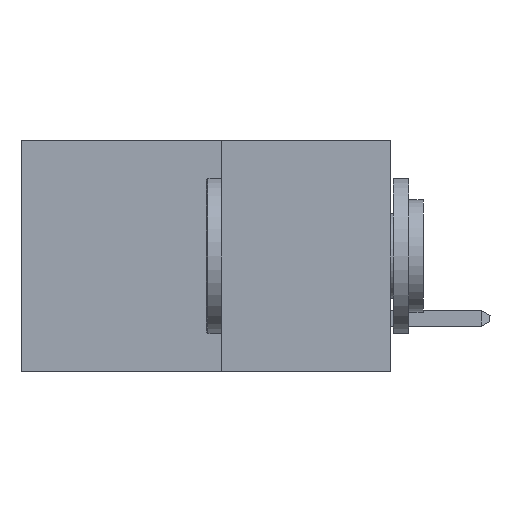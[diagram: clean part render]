
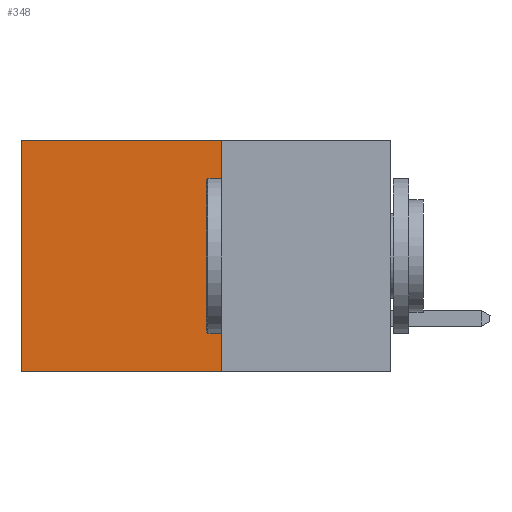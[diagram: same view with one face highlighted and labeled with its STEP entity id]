
A CAD part, left-side view. The second image highlights one B-rep face of the part: STEP entity #348.
In plain terms, the highlighted planar face has unit normal (-1, 0, 0).
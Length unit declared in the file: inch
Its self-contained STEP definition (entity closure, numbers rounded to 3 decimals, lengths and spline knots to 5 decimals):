
#348 = ADVANCED_FACE ( 'NONE', ( #4977 ), #7914, .F. ) ;
#482 = DIRECTION ( 'NONE',  ( 0., 1., 0. ) ) ;
#606 = DIRECTION ( 'NONE',  ( 0., 1., 0. ) ) ;
#948 = CARTESIAN_POINT ( 'NONE',  ( 0.277, 0.27, -0.37 ) ) ;
#1522 = EDGE_CURVE ( 'NONE', #10595, #3953, #10748, .T. ) ;
#2038 = CARTESIAN_POINT ( 'NONE',  ( 0.277, 0.59, -0.37 ) ) ;
#2112 = CARTESIAN_POINT ( 'NONE',  ( 0.277, 0.27, -0.37 ) ) ;
#2352 = CARTESIAN_POINT ( 'NONE',  ( 0.277, 0.59, 0. ) ) ;
#2364 = EDGE_CURVE ( 'NONE', #10306, #3953, #10005, .T. ) ;
#2389 = VECTOR ( 'NONE', #606, 39.37008 ) ;
#2398 = DIRECTION ( 'NONE',  ( 0., 0., -1. ) ) ;
#2627 = ORIENTED_EDGE ( 'NONE', *, *, #1522, .T. ) ;
#2659 = ORIENTED_EDGE ( 'NONE', *, *, #2873, .F. ) ;
#2672 = ORIENTED_EDGE ( 'NONE', *, *, #2364, .F. ) ;
#2873 = EDGE_CURVE ( 'NONE', #8517, #10306, #8238, .T. ) ;
#3453 = AXIS2_PLACEMENT_3D ( 'NONE', #9343, #8546, #4038 ) ;
#3911 = VECTOR ( 'NONE', #12240, 39.37008 ) ;
#3953 = VERTEX_POINT ( 'NONE', #4879 ) ;
#3961 = VECTOR ( 'NONE', #2398, 39.37008 ) ;
#4038 = DIRECTION ( 'NONE',  ( 0., 0., -1. ) ) ;
#4879 = CARTESIAN_POINT ( 'NONE',  ( 0.277, 0.59, -0.37 ) ) ;
#4882 = CARTESIAN_POINT ( 'NONE',  ( 0.277, 0.27, 0. ) ) ;
#4977 = FACE_OUTER_BOUND ( 'NONE', #8872, .T. ) ;
#7124 = EDGE_CURVE ( 'NONE', #8517, #10595, #8009, .T. ) ;
#7914 = PLANE ( 'NONE',  #3453 ) ;
#7918 = CARTESIAN_POINT ( 'NONE',  ( 0.277, 0.27, 0. ) ) ;
#8009 = LINE ( 'NONE', #4882, #12257 ) ;
#8238 = LINE ( 'NONE', #11873, #3911 ) ;
#8517 = VERTEX_POINT ( 'NONE', #7918 ) ;
#8546 = DIRECTION ( 'NONE',  ( 1., 0., 0. ) ) ;
#8809 = ORIENTED_EDGE ( 'NONE', *, *, #7124, .T. ) ;
#8872 = EDGE_LOOP ( 'NONE', ( #2627, #2672, #2659, #8809 ) ) ;
#9343 = CARTESIAN_POINT ( 'NONE',  ( 0.277, 0.27, -0.37 ) ) ;
#10005 = LINE ( 'NONE', #948, #2389 ) ;
#10306 = VERTEX_POINT ( 'NONE', #2112 ) ;
#10595 = VERTEX_POINT ( 'NONE', #2352 ) ;
#10748 = LINE ( 'NONE', #2038, #3961 ) ;
#11873 = CARTESIAN_POINT ( 'NONE',  ( 0.277, 0.27, -0.37 ) ) ;
#12240 = DIRECTION ( 'NONE',  ( 0., 0., -1. ) ) ;
#12257 = VECTOR ( 'NONE', #482, 39.37008 ) ;
